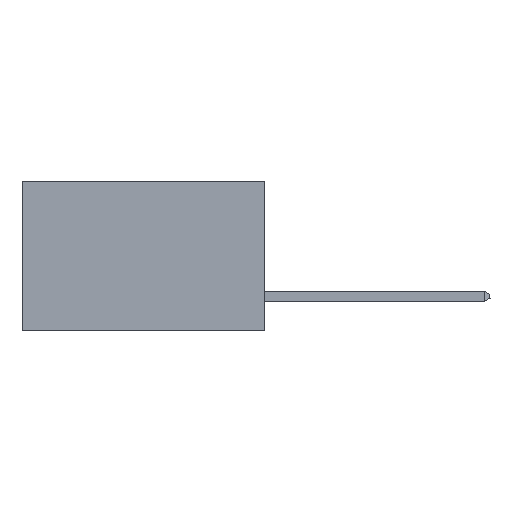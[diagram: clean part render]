
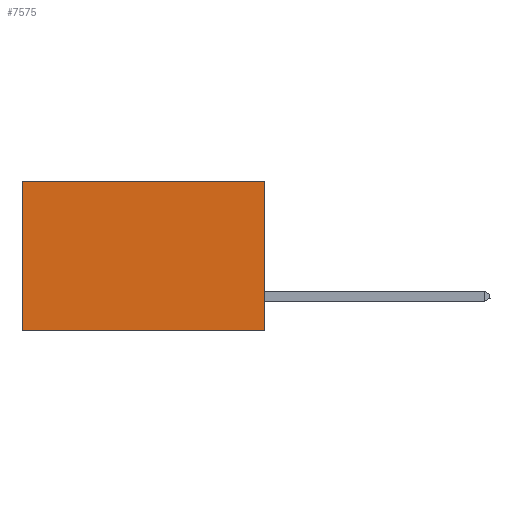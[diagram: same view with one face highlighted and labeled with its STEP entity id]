
A CAD part, left-side view. The second image highlights one B-rep face of the part: STEP entity #7575.
In plain terms, the highlighted planar face has unit normal (-1, 0, 0).
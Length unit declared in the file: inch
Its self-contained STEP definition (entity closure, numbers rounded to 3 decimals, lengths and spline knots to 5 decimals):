
#809 = VERTEX_POINT ( 'NONE', #14048 ) ;
#2266 = VERTEX_POINT ( 'NONE', #28542 ) ;
#3601 = VECTOR ( 'NONE', #8953, 39.37008 ) ;
#3725 = DIRECTION ( 'NONE',  ( 0., 0., -1. ) ) ;
#3849 = CARTESIAN_POINT ( 'NONE',  ( 0.298, 0.6, -0.37 ) ) ;
#5052 = CARTESIAN_POINT ( 'NONE',  ( 0.298, 0., 0. ) ) ;
#7134 = DIRECTION ( 'NONE',  ( 1., 0., 0. ) ) ;
#7575 = ADVANCED_FACE ( 'NONE', ( #12301 ), #18805, .F. ) ;
#8953 = DIRECTION ( 'NONE',  ( 0., 0., -1. ) ) ;
#9247 = ORIENTED_EDGE ( 'NONE', *, *, #22068, .F. ) ;
#9285 = EDGE_CURVE ( 'NONE', #13077, #809, #25864, .T. ) ;
#11310 = CARTESIAN_POINT ( 'NONE',  ( 0.298, 0., 0. ) ) ;
#12301 = FACE_OUTER_BOUND ( 'NONE', #14230, .T. ) ;
#13077 = VERTEX_POINT ( 'NONE', #11310 ) ;
#13302 = DIRECTION ( 'NONE',  ( 0., 1., 0. ) ) ;
#13358 = LINE ( 'NONE', #15794, #3601 ) ;
#13632 = VECTOR ( 'NONE', #13302, 39.37008 ) ;
#14048 = CARTESIAN_POINT ( 'NONE',  ( 0.298, 0.6, 0. ) ) ;
#14230 = EDGE_LOOP ( 'NONE', ( #27838, #9247, #25646, #23047 ) ) ;
#15301 = AXIS2_PLACEMENT_3D ( 'NONE', #5052, #7134, #19561 ) ;
#15794 = CARTESIAN_POINT ( 'NONE',  ( 0.298, 0., 0. ) ) ;
#15915 = CARTESIAN_POINT ( 'NONE',  ( 0.298, 0., -0.37 ) ) ;
#16221 = EDGE_CURVE ( 'NONE', #13077, #2266, #13358, .T. ) ;
#18437 = DIRECTION ( 'NONE',  ( 0., 1., 0. ) ) ;
#18805 = PLANE ( 'NONE',  #15301 ) ;
#19561 = DIRECTION ( 'NONE',  ( 0., 0., -1. ) ) ;
#20460 = LINE ( 'NONE', #24328, #27980 ) ;
#21327 = VECTOR ( 'NONE', #18437, 39.37008 ) ;
#22068 = EDGE_CURVE ( 'NONE', #2266, #24573, #27050, .T. ) ;
#22242 = CARTESIAN_POINT ( 'NONE',  ( 0.298, 0., 0. ) ) ;
#23047 = ORIENTED_EDGE ( 'NONE', *, *, #9285, .T. ) ;
#24328 = CARTESIAN_POINT ( 'NONE',  ( 0.298, 0.6, 0. ) ) ;
#24573 = VERTEX_POINT ( 'NONE', #3849 ) ;
#25646 = ORIENTED_EDGE ( 'NONE', *, *, #16221, .F. ) ;
#25864 = LINE ( 'NONE', #22242, #13632 ) ;
#26199 = EDGE_CURVE ( 'NONE', #809, #24573, #20460, .T. ) ;
#27050 = LINE ( 'NONE', #15915, #21327 ) ;
#27838 = ORIENTED_EDGE ( 'NONE', *, *, #26199, .T. ) ;
#27980 = VECTOR ( 'NONE', #3725, 39.37008 ) ;
#28542 = CARTESIAN_POINT ( 'NONE',  ( 0.298, 0., -0.37 ) ) ;
